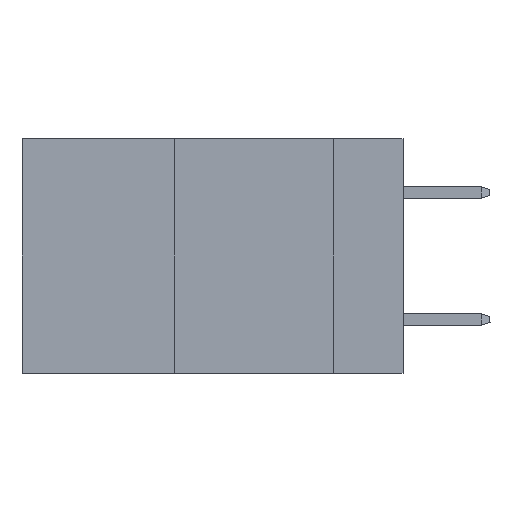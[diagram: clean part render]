
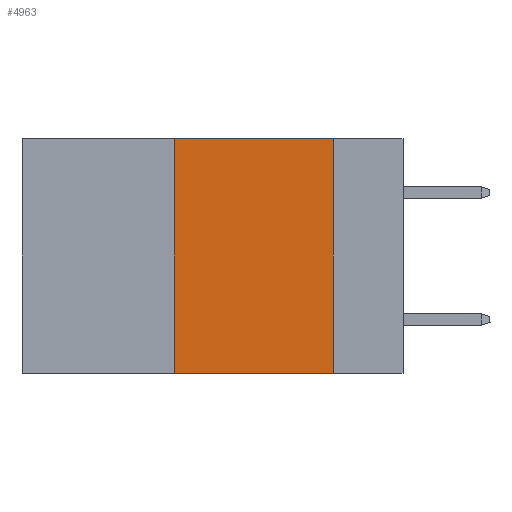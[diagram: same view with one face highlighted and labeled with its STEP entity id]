
A CAD part, left-side view. The second image highlights one B-rep face of the part: STEP entity #4963.
In plain terms, the highlighted planar face has unit normal (-1, 0, 0).
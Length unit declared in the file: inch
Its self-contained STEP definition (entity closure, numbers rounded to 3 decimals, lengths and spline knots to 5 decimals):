
#412 = ORIENTED_EDGE ( 'NONE', *, *, #3314, .F. ) ;
#651 = VERTEX_POINT ( 'NONE', #2523 ) ;
#1659 = AXIS2_PLACEMENT_3D ( 'NONE', #14022, #20667, #12319 ) ;
#1782 = CARTESIAN_POINT ( 'NONE',  ( 0., 0.11, -0.37 ) ) ;
#2335 = CARTESIAN_POINT ( 'NONE',  ( 0., 0.36, -0.37 ) ) ;
#2523 = CARTESIAN_POINT ( 'NONE',  ( 0., 0.11, 0. ) ) ;
#2591 = PLANE ( 'NONE',  #1659 ) ;
#2605 = CARTESIAN_POINT ( 'NONE',  ( 0., 0.6, 0. ) ) ;
#3314 = EDGE_CURVE ( 'NONE', #5330, #6551, #6387, .T. ) ;
#4425 = LINE ( 'NONE', #11069, #7358 ) ;
#4599 = DIRECTION ( 'NONE',  ( 0., -1., 0. ) ) ;
#4882 = CARTESIAN_POINT ( 'NONE',  ( 0., 0.36, 0. ) ) ;
#4963 = ADVANCED_FACE ( 'NONE', ( #17428 ), #2591, .F. ) ;
#5330 = VERTEX_POINT ( 'NONE', #2335 ) ;
#5394 = CARTESIAN_POINT ( 'NONE',  ( 0., 0.36, 0. ) ) ;
#6387 = LINE ( 'NONE', #4882, #12409 ) ;
#6551 = VERTEX_POINT ( 'NONE', #5394 ) ;
#6823 = ORIENTED_EDGE ( 'NONE', *, *, #12347, .F. ) ;
#7358 = VECTOR ( 'NONE', #7467, 39.37008 ) ;
#7467 = DIRECTION ( 'NONE',  ( 0., -1., 0. ) ) ;
#7695 = CARTESIAN_POINT ( 'NONE',  ( 0., 0.11, 0. ) ) ;
#7732 = LINE ( 'NONE', #2605, #10845 ) ;
#7774 = EDGE_CURVE ( 'NONE', #5330, #14952, #4425, .T. ) ;
#7810 = LINE ( 'NONE', #7695, #18476 ) ;
#7919 = DIRECTION ( 'NONE',  ( 0., 0., -1. ) ) ;
#10845 = VECTOR ( 'NONE', #4599, 39.37008 ) ;
#11069 = CARTESIAN_POINT ( 'NONE',  ( 0., 0.6, -0.37 ) ) ;
#12319 = DIRECTION ( 'NONE',  ( 0., 0., -1. ) ) ;
#12347 = EDGE_CURVE ( 'NONE', #651, #14952, #7810, .T. ) ;
#12409 = VECTOR ( 'NONE', #17960, 39.37008 ) ;
#14022 = CARTESIAN_POINT ( 'NONE',  ( 0., 0.6, 0. ) ) ;
#14952 = VERTEX_POINT ( 'NONE', #1782 ) ;
#16356 = ORIENTED_EDGE ( 'NONE', *, *, #7774, .T. ) ;
#17428 = FACE_OUTER_BOUND ( 'NONE', #20966, .T. ) ;
#17960 = DIRECTION ( 'NONE',  ( 0., 0., 1. ) ) ;
#18476 = VECTOR ( 'NONE', #7919, 39.37008 ) ;
#19889 = ORIENTED_EDGE ( 'NONE', *, *, #20001, .F. ) ;
#20001 = EDGE_CURVE ( 'NONE', #6551, #651, #7732, .T. ) ;
#20667 = DIRECTION ( 'NONE',  ( 1., 0., 0. ) ) ;
#20966 = EDGE_LOOP ( 'NONE', ( #6823, #19889, #412, #16356 ) ) ;
